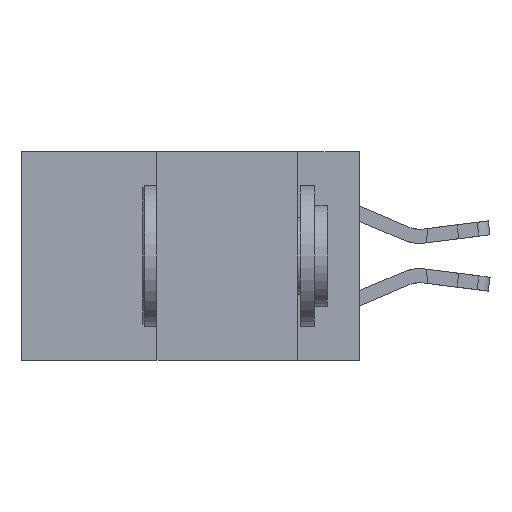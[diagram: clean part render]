
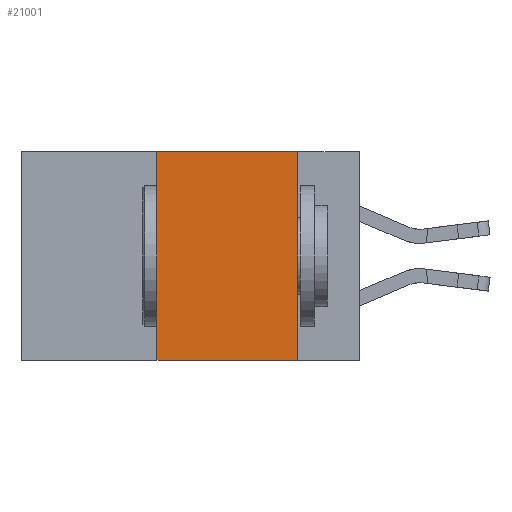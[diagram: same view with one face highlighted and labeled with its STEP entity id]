
A CAD part, left-side view. The second image highlights one B-rep face of the part: STEP entity #21001.
In plain terms, the highlighted planar face has unit normal (-1, 0, 0).
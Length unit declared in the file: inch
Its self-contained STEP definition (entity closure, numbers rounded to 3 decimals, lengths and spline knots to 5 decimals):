
#520 = VECTOR ( 'NONE', #20053, 39.37008 ) ;
#1165 = LINE ( 'NONE', #16144, #520 ) ;
#4043 = LINE ( 'NONE', #9590, #14272 ) ;
#4683 = AXIS2_PLACEMENT_3D ( 'NONE', #21532, #23532, #25581 ) ;
#6733 = LINE ( 'NONE', #21500, #16891 ) ;
#8358 = VERTEX_POINT ( 'NONE', #19851 ) ;
#8960 = LINE ( 'NONE', #10438, #14072 ) ;
#9590 = CARTESIAN_POINT ( 'NONE',  ( 0., 0.11, 0. ) ) ;
#10183 = FACE_OUTER_BOUND ( 'NONE', #22392, .T. ) ;
#10438 = CARTESIAN_POINT ( 'NONE',  ( 0., 0.6, 0. ) ) ;
#14072 = VECTOR ( 'NONE', #20705, 39.37008 ) ;
#14143 = CARTESIAN_POINT ( 'NONE',  ( 0., 0.36, -0.37 ) ) ;
#14272 = VECTOR ( 'NONE', #21639, 39.37008 ) ;
#16144 = CARTESIAN_POINT ( 'NONE',  ( 0., 0.6, -0.37 ) ) ;
#16428 = ORIENTED_EDGE ( 'NONE', *, *, #19862, .F. ) ;
#16464 = VERTEX_POINT ( 'NONE', #14143 ) ;
#16466 = CARTESIAN_POINT ( 'NONE',  ( 0., 0.36, 0. ) ) ;
#16891 = VECTOR ( 'NONE', #18455, 39.37008 ) ;
#17629 = ORIENTED_EDGE ( 'NONE', *, *, #22644, .T. ) ;
#18455 = DIRECTION ( 'NONE',  ( 0., 0., 1. ) ) ;
#19851 = CARTESIAN_POINT ( 'NONE',  ( 0., 0.11, 0. ) ) ;
#19862 = EDGE_CURVE ( 'NONE', #16464, #22884, #6733, .T. ) ;
#20053 = DIRECTION ( 'NONE',  ( 0., -1., 0. ) ) ;
#20503 = ORIENTED_EDGE ( 'NONE', *, *, #25902, .F. ) ;
#20705 = DIRECTION ( 'NONE',  ( 0., -1., 0. ) ) ;
#20727 = VERTEX_POINT ( 'NONE', #24271 ) ;
#21001 = ADVANCED_FACE ( 'NONE', ( #10183 ), #25489, .F. ) ;
#21500 = CARTESIAN_POINT ( 'NONE',  ( 0., 0.36, 0. ) ) ;
#21532 = CARTESIAN_POINT ( 'NONE',  ( 0., 0.6, 0. ) ) ;
#21639 = DIRECTION ( 'NONE',  ( 0., 0., -1. ) ) ;
#22128 = EDGE_CURVE ( 'NONE', #8358, #20727, #4043, .T. ) ;
#22392 = EDGE_LOOP ( 'NONE', ( #25985, #20503, #16428, #17629 ) ) ;
#22644 = EDGE_CURVE ( 'NONE', #16464, #20727, #1165, .T. ) ;
#22884 = VERTEX_POINT ( 'NONE', #16466 ) ;
#23532 = DIRECTION ( 'NONE',  ( 1., 0., 0. ) ) ;
#24271 = CARTESIAN_POINT ( 'NONE',  ( 0., 0.11, -0.37 ) ) ;
#25489 = PLANE ( 'NONE',  #4683 ) ;
#25581 = DIRECTION ( 'NONE',  ( 0., 0., -1. ) ) ;
#25902 = EDGE_CURVE ( 'NONE', #22884, #8358, #8960, .T. ) ;
#25985 = ORIENTED_EDGE ( 'NONE', *, *, #22128, .F. ) ;
